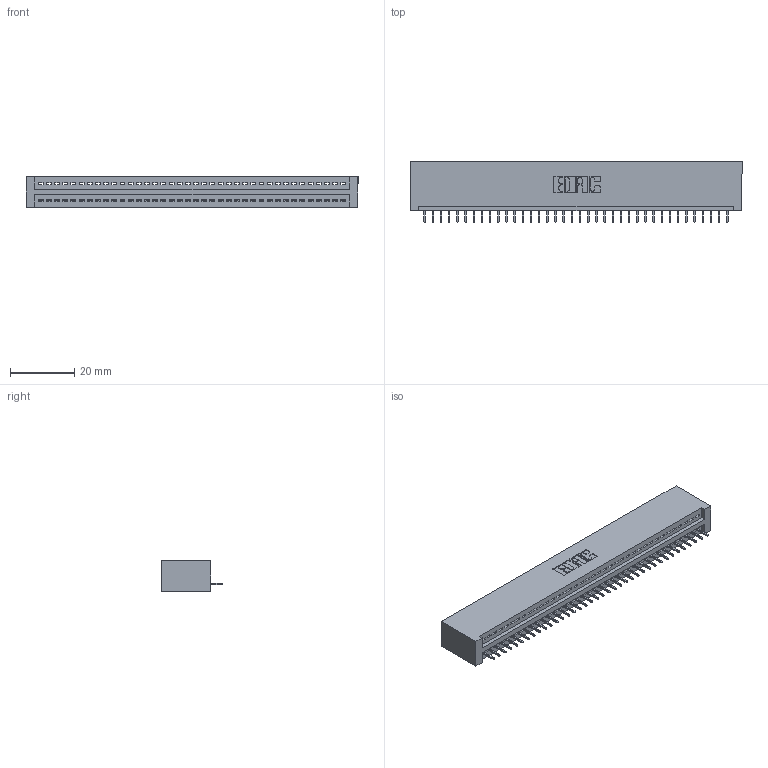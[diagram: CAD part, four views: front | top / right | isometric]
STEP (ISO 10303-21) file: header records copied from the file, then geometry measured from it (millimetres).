
FILE_DESCRIPTION (( 'STEP AP203' ), '1' );
FILE_NAME ('345-038-525-101.STEP', '2020-09-19T17:37:41', ( '' ), ( '' ), 'SwSTEP 2.0', 'SolidWorks 2020', '' );
FILE_SCHEMA (( 'CONFIG_CONTROL_DESIGN' ));
Length unit declared in the file: inch
Products named in the file (3): 345-292-001_345-293-125; 345-038-525-101; 345 Part_No Mounting Lugs
Assembly tree (39 placements, depth 2):
  345-038-525-101
    345 Part_No Mounting Lugs
    345-292-001_345-293-125  x38
Bounding box: 103.12 x 18.72 x 9.4 mm (x, y, z)
Volume: 10191.3 mm3; surface area: 13161.7 mm2
Topology: 39 solids, 39 shells, 2474 faces, 7157 edges, 4618 vertices
Faces by surface type: plane 1824, cylinder 650
Entity records: 28935 total; most frequent: CARTESIAN_POINT 5018, ORIENTED_EDGE 4990, DIRECTION 4383, EDGE_CURVE 2495, VECTOR 2223, LINE 2223, VERTEX_POINT 1658, AXIS2_PLACEMENT_3D 1080
